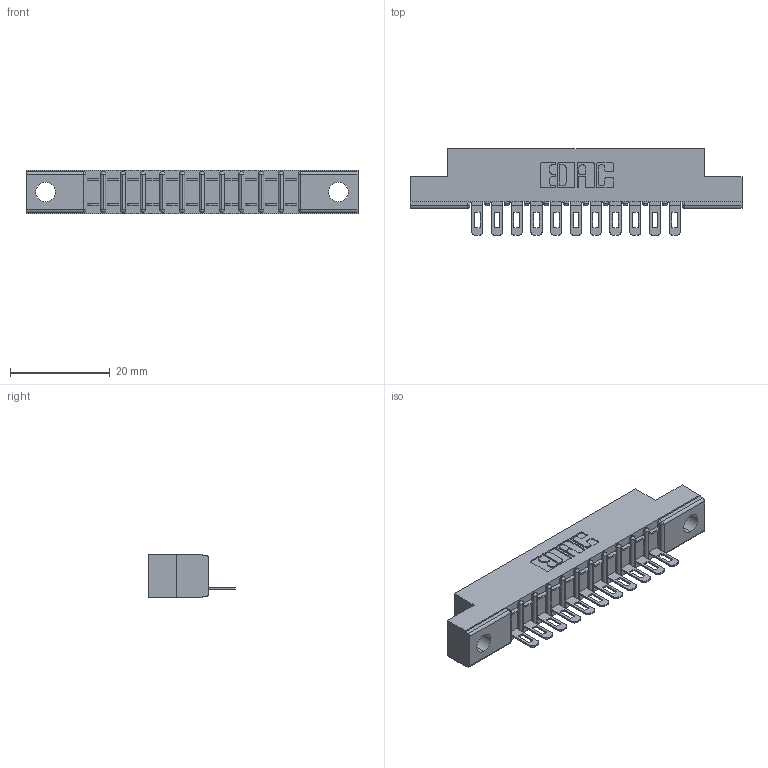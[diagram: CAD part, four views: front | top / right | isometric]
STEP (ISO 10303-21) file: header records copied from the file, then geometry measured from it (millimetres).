
FILE_DESCRIPTION (( 'STEP AP203' ), '1' );
FILE_NAME ('307-011-501-104.STEP', '2019-09-04T19:22:02', ( '' ), ( '' ), 'SwSTEP 2.0', 'SolidWorks 2016', '' );
FILE_SCHEMA (( 'CONFIG_CONTROL_DESIGN' ));
Length unit declared in the file: inch
Products named in the file (3): 307-290-002_501; 307-011-501-104; 307 Part_.156 Dia Mounting Holes
Assembly tree (12 placements, depth 2):
  307-011-501-104
    307 Part_.156 Dia Mounting Holes
    307-290-002_501  x11
Bounding box: 66.6 x 17.42 x 8.71 mm (x, y, z)
Volume: 4294.6 mm3; surface area: 7164.3 mm2
Topology: 12 solids, 12 shells, 980 faces, 2977 edges, 1950 vertices
Faces by surface type: plane 568, cylinder 388, sphere 24
Entity records: 14464 total; most frequent: CARTESIAN_POINT 2438, ORIENTED_EDGE 2426, DIRECTION 2379, EDGE_CURVE 1213, VECTOR 917, LINE 917, VERTEX_POINT 790, AXIS2_PLACEMENT_3D 731
